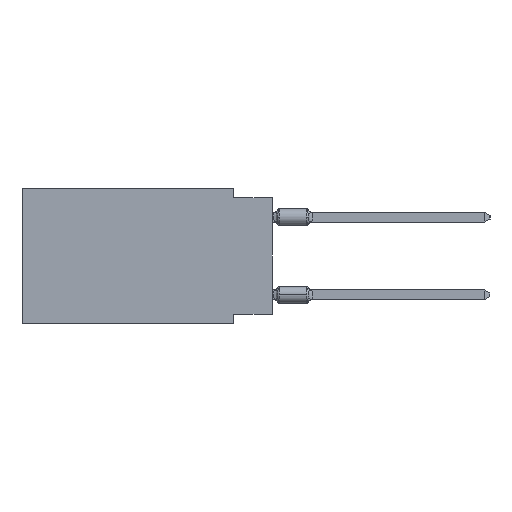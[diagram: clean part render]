
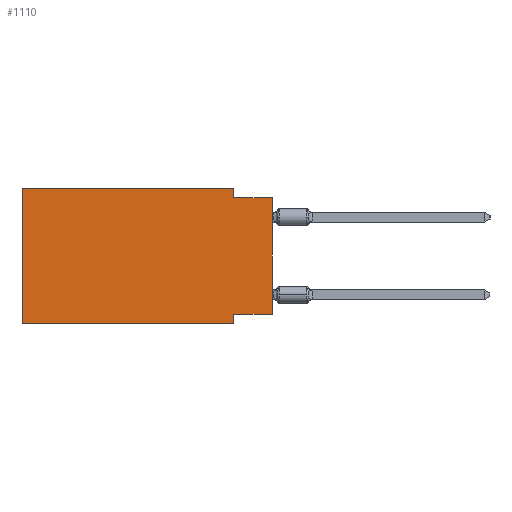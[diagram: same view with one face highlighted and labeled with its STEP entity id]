
A CAD part, left-side view. The second image highlights one B-rep face of the part: STEP entity #1110.
In plain terms, the highlighted planar face has unit normal (-1, 0, 0).
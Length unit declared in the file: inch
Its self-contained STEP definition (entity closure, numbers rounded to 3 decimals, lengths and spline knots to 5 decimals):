
#234 = CARTESIAN_POINT ( 'NONE',  ( 0., 0.1, -0.35 ) ) ;
#628 = FACE_OUTER_BOUND ( 'NONE', #26374, .T. ) ;
#1110 = ADVANCED_FACE ( 'NONE', ( #628 ), #4300, .F. ) ;
#1631 = ORIENTED_EDGE ( 'NONE', *, *, #10433, .F. ) ;
#2019 = CARTESIAN_POINT ( 'NONE',  ( 0., 0., -0.325 ) ) ;
#2498 = LINE ( 'NONE', #2019, #37646 ) ;
#4300 = PLANE ( 'NONE',  #38559 ) ;
#4466 = DIRECTION ( 'NONE',  ( 0., 0., -1. ) ) ;
#4624 = VECTOR ( 'NONE', #35288, 39.37008 ) ;
#5300 = VECTOR ( 'NONE', #12488, 39.37008 ) ;
#5896 = CARTESIAN_POINT ( 'NONE',  ( 0., 0., -0.325 ) ) ;
#6207 = EDGE_CURVE ( 'NONE', #17368, #26617, #11147, .T. ) ;
#6551 = VERTEX_POINT ( 'NONE', #9418 ) ;
#7331 = ORIENTED_EDGE ( 'NONE', *, *, #45559, .F. ) ;
#7839 = CARTESIAN_POINT ( 'NONE',  ( 0., 0.1, 0. ) ) ;
#7908 = LINE ( 'NONE', #30892, #46674 ) ;
#9418 = CARTESIAN_POINT ( 'NONE',  ( 0., 0.645, -0.35 ) ) ;
#9979 = LINE ( 'NONE', #39826, #40579 ) ;
#10090 = DIRECTION ( 'NONE',  ( 0., 1., 0. ) ) ;
#10433 = EDGE_CURVE ( 'NONE', #14201, #32482, #7908, .T. ) ;
#11147 = LINE ( 'NONE', #44679, #41397 ) ;
#12488 = DIRECTION ( 'NONE',  ( 0., -1., 0. ) ) ;
#14201 = VERTEX_POINT ( 'NONE', #27696 ) ;
#14225 = VERTEX_POINT ( 'NONE', #5896 ) ;
#14378 = ORIENTED_EDGE ( 'NONE', *, *, #43700, .T. ) ;
#16891 = CARTESIAN_POINT ( 'NONE',  ( 0., 0.645, -0.35 ) ) ;
#17368 = VERTEX_POINT ( 'NONE', #36319 ) ;
#17815 = EDGE_CURVE ( 'NONE', #14225, #30460, #46328, .T. ) ;
#18751 = DIRECTION ( 'NONE',  ( 1., 0., 0. ) ) ;
#19283 = ORIENTED_EDGE ( 'NONE', *, *, #6207, .F. ) ;
#19469 = DIRECTION ( 'NONE',  ( 0., 0., -1. ) ) ;
#19678 = EDGE_CURVE ( 'NONE', #26617, #25205, #21185, .T. ) ;
#20104 = CARTESIAN_POINT ( 'NONE',  ( 0., 0., 0. ) ) ;
#20736 = DIRECTION ( 'NONE',  ( 0., 0., 1. ) ) ;
#21185 = LINE ( 'NONE', #33158, #46164 ) ;
#21860 = VECTOR ( 'NONE', #36213, 39.37008 ) ;
#23492 = LINE ( 'NONE', #38442, #5300 ) ;
#25205 = VERTEX_POINT ( 'NONE', #41897 ) ;
#26374 = EDGE_LOOP ( 'NONE', ( #29963, #29309, #45750, #19283, #33726, #14378, #1631, #7331 ) ) ;
#26617 = VERTEX_POINT ( 'NONE', #7839 ) ;
#27696 = CARTESIAN_POINT ( 'NONE',  ( 0., 0.1, -0.325 ) ) ;
#29309 = ORIENTED_EDGE ( 'NONE', *, *, #41223, .F. ) ;
#29603 = CARTESIAN_POINT ( 'NONE',  ( 0., 0., -0.025 ) ) ;
#29963 = ORIENTED_EDGE ( 'NONE', *, *, #17815, .T. ) ;
#30460 = VERTEX_POINT ( 'NONE', #29603 ) ;
#30892 = CARTESIAN_POINT ( 'NONE',  ( 0., 0.1, -0.35 ) ) ;
#32482 = VERTEX_POINT ( 'NONE', #234 ) ;
#33158 = CARTESIAN_POINT ( 'NONE',  ( 0., 0.1, 0. ) ) ;
#33726 = ORIENTED_EDGE ( 'NONE', *, *, #42919, .F. ) ;
#35288 = DIRECTION ( 'NONE',  ( 0., 0., 1. ) ) ;
#36128 = DIRECTION ( 'NONE',  ( 0., 0., -1. ) ) ;
#36213 = DIRECTION ( 'NONE',  ( 0., -1., 0. ) ) ;
#36319 = CARTESIAN_POINT ( 'NONE',  ( 0., 0.645, 0. ) ) ;
#37646 = VECTOR ( 'NONE', #10090, 39.37008 ) ;
#38442 = CARTESIAN_POINT ( 'NONE',  ( 0., 0., -0.025 ) ) ;
#38559 = AXIS2_PLACEMENT_3D ( 'NONE', #45677, #18751, #19469 ) ;
#39826 = CARTESIAN_POINT ( 'NONE',  ( 0., 0.645, 0. ) ) ;
#40517 = DIRECTION ( 'NONE',  ( 0., -1., 0. ) ) ;
#40579 = VECTOR ( 'NONE', #20736, 39.37008 ) ;
#41223 = EDGE_CURVE ( 'NONE', #25205, #30460, #23492, .T. ) ;
#41397 = VECTOR ( 'NONE', #40517, 39.37008 ) ;
#41897 = CARTESIAN_POINT ( 'NONE',  ( 0., 0.1, -0.025 ) ) ;
#42919 = EDGE_CURVE ( 'NONE', #6551, #17368, #9979, .T. ) ;
#43700 = EDGE_CURVE ( 'NONE', #6551, #32482, #47243, .T. ) ;
#44679 = CARTESIAN_POINT ( 'NONE',  ( 0., 0.645, 0. ) ) ;
#45559 = EDGE_CURVE ( 'NONE', #14225, #14201, #2498, .T. ) ;
#45677 = CARTESIAN_POINT ( 'NONE',  ( 0., 0.645, 0. ) ) ;
#45750 = ORIENTED_EDGE ( 'NONE', *, *, #19678, .F. ) ;
#46164 = VECTOR ( 'NONE', #36128, 39.37008 ) ;
#46328 = LINE ( 'NONE', #20104, #4624 ) ;
#46674 = VECTOR ( 'NONE', #4466, 39.37008 ) ;
#47243 = LINE ( 'NONE', #16891, #21860 ) ;
